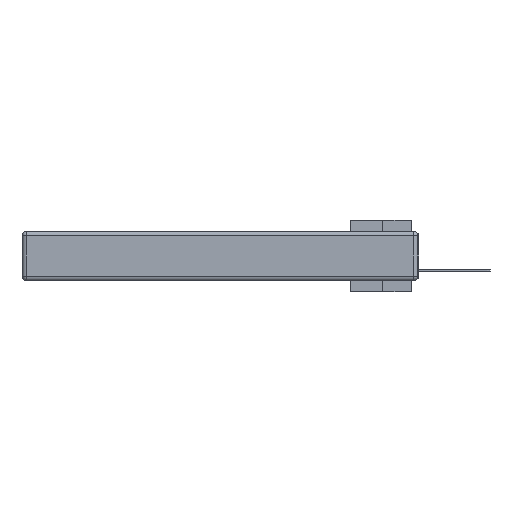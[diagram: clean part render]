
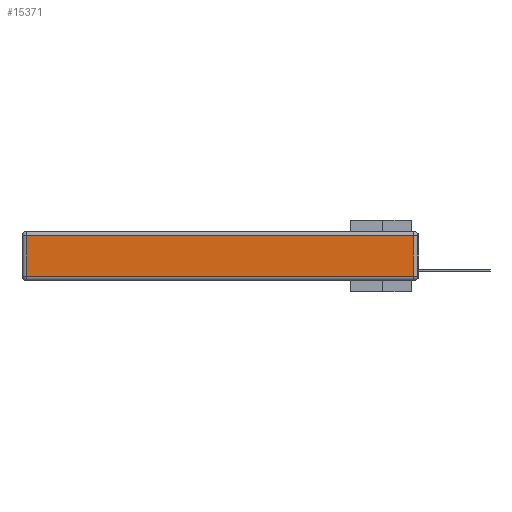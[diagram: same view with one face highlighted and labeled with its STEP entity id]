
A CAD part, left-side view. The second image highlights one B-rep face of the part: STEP entity #15371.
In plain terms, the highlighted planar face has unit normal (-1, 0, 0).
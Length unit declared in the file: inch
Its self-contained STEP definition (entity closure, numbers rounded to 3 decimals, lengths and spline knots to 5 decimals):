
#278 = EDGE_CURVE ( 'NONE', #23761, #17273, #25406, .T. ) ;
#575 = CARTESIAN_POINT ( 'NONE',  ( 0., 2.75, -0.03 ) ) ;
#1693 = CARTESIAN_POINT ( 'NONE',  ( 0., 2.72, -0.343 ) ) ;
#2191 = VECTOR ( 'NONE', #26983, 39.37008 ) ;
#2260 = CARTESIAN_POINT ( 'NONE',  ( 0., 0.03, -0.03 ) ) ;
#2976 = EDGE_CURVE ( 'NONE', #13253, #14343, #12882, .T. ) ;
#3457 = EDGE_CURVE ( 'NONE', #17273, #13253, #17957, .T. ) ;
#4000 = DIRECTION ( 'NONE',  ( 0., 0., 1. ) ) ;
#4413 = ORIENTED_EDGE ( 'NONE', *, *, #278, .T. ) ;
#5178 = EDGE_LOOP ( 'NONE', ( #22174, #8448, #26264, #4413 ) ) ;
#7000 = CARTESIAN_POINT ( 'NONE',  ( 0., 0., -0.343 ) ) ;
#8448 = ORIENTED_EDGE ( 'NONE', *, *, #2976, .T. ) ;
#10842 = CARTESIAN_POINT ( 'NONE',  ( 0., 2.72, -0.313 ) ) ;
#11127 = CARTESIAN_POINT ( 'NONE',  ( 0., 0.03, -0.343 ) ) ;
#11203 = DIRECTION ( 'NONE',  ( 0., 0., 1. ) ) ;
#12882 = LINE ( 'NONE', #11127, #23054 ) ;
#13192 = VECTOR ( 'NONE', #16845, 39.37008 ) ;
#13253 = VERTEX_POINT ( 'NONE', #22223 ) ;
#14343 = VERTEX_POINT ( 'NONE', #2260 ) ;
#15158 = EDGE_CURVE ( 'NONE', #14343, #23761, #18600, .T. ) ;
#15371 = ADVANCED_FACE ( 'NONE', ( #26186 ), #27723, .T. ) ;
#16804 = VECTOR ( 'NONE', #27524, 39.37008 ) ;
#16845 = DIRECTION ( 'NONE',  ( 0., 1., 0. ) ) ;
#17273 = VERTEX_POINT ( 'NONE', #10842 ) ;
#17957 = LINE ( 'NONE', #20593, #16804 ) ;
#18600 = LINE ( 'NONE', #575, #13192 ) ;
#20593 = CARTESIAN_POINT ( 'NONE',  ( 0., 0., -0.313 ) ) ;
#22174 = ORIENTED_EDGE ( 'NONE', *, *, #3457, .T. ) ;
#22223 = CARTESIAN_POINT ( 'NONE',  ( 0., 0.03, -0.313 ) ) ;
#23054 = VECTOR ( 'NONE', #4000, 39.37008 ) ;
#23216 = DIRECTION ( 'NONE',  ( -1., 0., 0. ) ) ;
#23761 = VERTEX_POINT ( 'NONE', #24261 ) ;
#24261 = CARTESIAN_POINT ( 'NONE',  ( 0., 2.72, -0.03 ) ) ;
#25406 = LINE ( 'NONE', #1693, #2191 ) ;
#26186 = FACE_OUTER_BOUND ( 'NONE', #5178, .T. ) ;
#26264 = ORIENTED_EDGE ( 'NONE', *, *, #15158, .T. ) ;
#26983 = DIRECTION ( 'NONE',  ( 0., 0., -1. ) ) ;
#27524 = DIRECTION ( 'NONE',  ( 0., -1., 0. ) ) ;
#27526 = AXIS2_PLACEMENT_3D ( 'NONE', #7000, #23216, #11203 ) ;
#27723 = PLANE ( 'NONE',  #27526 ) ;
